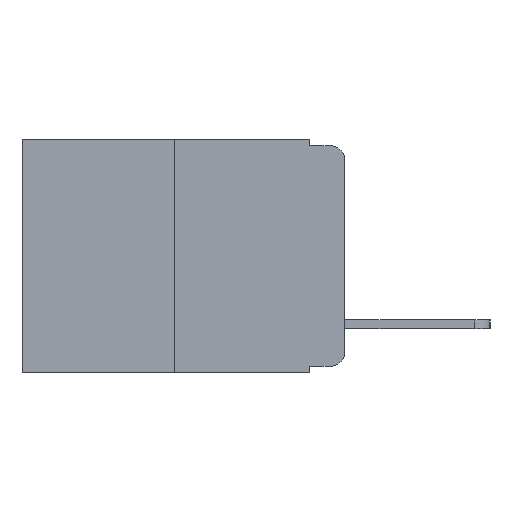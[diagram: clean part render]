
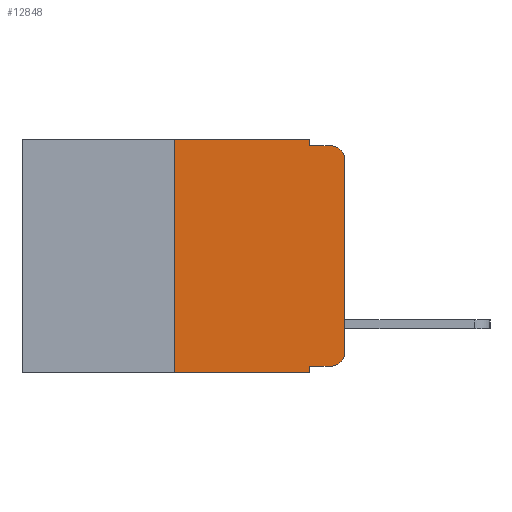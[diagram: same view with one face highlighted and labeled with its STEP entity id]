
A CAD part, left-side view. The second image highlights one B-rep face of the part: STEP entity #12848.
In plain terms, the highlighted planar face has unit normal (-1, 0, 0).
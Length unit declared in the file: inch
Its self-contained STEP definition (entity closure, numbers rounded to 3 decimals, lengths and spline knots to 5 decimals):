
#46 = ORIENTED_EDGE ( 'NONE', *, *, #10113, .T. ) ;
#92 = VECTOR ( 'NONE', #14581, 39.37008 ) ;
#102 = DIRECTION ( 'NONE',  ( 1., 0., 0. ) ) ;
#132 = CARTESIAN_POINT ( 'NONE',  ( 0., 0.02, -0.313 ) ) ;
#219 = VERTEX_POINT ( 'NONE', #14642 ) ;
#473 = CARTESIAN_POINT ( 'NONE',  ( 0., 0., -0.03 ) ) ;
#903 = VECTOR ( 'NONE', #10060, 39.37008 ) ;
#1251 = VERTEX_POINT ( 'NONE', #1979 ) ;
#1410 = EDGE_CURVE ( 'NONE', #9491, #15023, #4073, .T. ) ;
#1529 = DIRECTION ( 'NONE',  ( 0., 0., -1. ) ) ;
#1979 = CARTESIAN_POINT ( 'NONE',  ( 0., 0.25, -0.343 ) ) ;
#2309 = EDGE_CURVE ( 'NONE', #9491, #8995, #4041, .T. ) ;
#2317 = DIRECTION ( 'NONE',  ( 0., -1., 0. ) ) ;
#2526 = FACE_OUTER_BOUND ( 'NONE', #15947, .T. ) ;
#2939 = ORIENTED_EDGE ( 'NONE', *, *, #16074, .T. ) ;
#3181 = EDGE_CURVE ( 'NONE', #1251, #8301, #5237, .T. ) ;
#3269 = AXIS2_PLACEMENT_3D ( 'NONE', #12316, #4678, #13518 ) ;
#3487 = ORIENTED_EDGE ( 'NONE', *, *, #7555, .F. ) ;
#3507 = ORIENTED_EDGE ( 'NONE', *, *, #4931, .F. ) ;
#3775 = LINE ( 'NONE', #3844, #13476 ) ;
#3844 = CARTESIAN_POINT ( 'NONE',  ( 0., 0.051, -0.01 ) ) ;
#4041 = LINE ( 'NONE', #13116, #13716 ) ;
#4073 = LINE ( 'NONE', #10340, #92 ) ;
#4083 = CARTESIAN_POINT ( 'NONE',  ( 0., 0.473, 0. ) ) ;
#4241 = ORIENTED_EDGE ( 'NONE', *, *, #9272, .T. ) ;
#4269 = CIRCLE ( 'NONE', #10270, 0.02 ) ;
#4285 = AXIS2_PLACEMENT_3D ( 'NONE', #4083, #102, #9298 ) ;
#4678 = DIRECTION ( 'NONE',  ( -1., 0., 0. ) ) ;
#4692 = VECTOR ( 'NONE', #2317, 39.37008 ) ;
#4822 = VERTEX_POINT ( 'NONE', #9692 ) ;
#4849 = ORIENTED_EDGE ( 'NONE', *, *, #2309, .F. ) ;
#4856 = CARTESIAN_POINT ( 'NONE',  ( 0., 0.02, -0.01 ) ) ;
#4931 = EDGE_CURVE ( 'NONE', #219, #9879, #4998, .T. ) ;
#4998 = LINE ( 'NONE', #15694, #8429 ) ;
#5237 = LINE ( 'NONE', #15120, #903 ) ;
#5469 = DIRECTION ( 'NONE',  ( 0., -1., 0. ) ) ;
#5485 = ORIENTED_EDGE ( 'NONE', *, *, #16097, .F. ) ;
#5561 = ORIENTED_EDGE ( 'NONE', *, *, #3181, .F. ) ;
#5907 = CARTESIAN_POINT ( 'NONE',  ( 0., 0.02, -0.333 ) ) ;
#6093 = VECTOR ( 'NONE', #5469, 39.37008 ) ;
#6770 = CIRCLE ( 'NONE', #3269, 0.02 ) ;
#7018 = CARTESIAN_POINT ( 'NONE',  ( 0., 0.25, 0. ) ) ;
#7090 = DIRECTION ( 'NONE',  ( 0., 0., -1. ) ) ;
#7145 = CARTESIAN_POINT ( 'NONE',  ( 0., 0.051, -0.01 ) ) ;
#7507 = DIRECTION ( 'NONE',  ( 0., 0., -1. ) ) ;
#7555 = EDGE_CURVE ( 'NONE', #9879, #9377, #3775, .T. ) ;
#7561 = VECTOR ( 'NONE', #8985, 39.37008 ) ;
#7589 = ORIENTED_EDGE ( 'NONE', *, *, #15168, .T. ) ;
#7991 = PLANE ( 'NONE',  #4285 ) ;
#8301 = VERTEX_POINT ( 'NONE', #7018 ) ;
#8429 = VECTOR ( 'NONE', #7090, 39.37008 ) ;
#8985 = DIRECTION ( 'NONE',  ( 0., 0., 1. ) ) ;
#8995 = VERTEX_POINT ( 'NONE', #16280 ) ;
#9272 = EDGE_CURVE ( 'NONE', #13026, #9377, #6770, .T. ) ;
#9298 = DIRECTION ( 'NONE',  ( 0., 0., -1. ) ) ;
#9321 = DIRECTION ( 'NONE',  ( -1., 0., 0. ) ) ;
#9377 = VERTEX_POINT ( 'NONE', #4856 ) ;
#9491 = VERTEX_POINT ( 'NONE', #11477 ) ;
#9535 = LINE ( 'NONE', #14224, #6093 ) ;
#9692 = CARTESIAN_POINT ( 'NONE',  ( 0., 0., -0.313 ) ) ;
#9879 = VERTEX_POINT ( 'NONE', #7145 ) ;
#10060 = DIRECTION ( 'NONE',  ( 0., 0., 1. ) ) ;
#10067 = CARTESIAN_POINT ( 'NONE',  ( 0., 0.473, -0.343 ) ) ;
#10113 = EDGE_CURVE ( 'NONE', #4822, #13026, #10942, .T. ) ;
#10270 = AXIS2_PLACEMENT_3D ( 'NONE', #132, #9321, #1529 ) ;
#10340 = CARTESIAN_POINT ( 'NONE',  ( 0., 0.051, -0.333 ) ) ;
#10807 = ORIENTED_EDGE ( 'NONE', *, *, #1410, .T. ) ;
#10942 = LINE ( 'NONE', #16249, #7561 ) ;
#11477 = CARTESIAN_POINT ( 'NONE',  ( 0., 0.051, -0.333 ) ) ;
#11530 = LINE ( 'NONE', #10067, #4692 ) ;
#11534 = DIRECTION ( 'NONE',  ( 0., -1., 0. ) ) ;
#12316 = CARTESIAN_POINT ( 'NONE',  ( 0., 0.02, -0.03 ) ) ;
#12848 = ADVANCED_FACE ( 'NONE', ( #2526 ), #7991, .F. ) ;
#13026 = VERTEX_POINT ( 'NONE', #473 ) ;
#13116 = CARTESIAN_POINT ( 'NONE',  ( 0., 0.051, 0. ) ) ;
#13476 = VECTOR ( 'NONE', #11534, 39.37008 ) ;
#13518 = DIRECTION ( 'NONE',  ( 0., 0., -1. ) ) ;
#13716 = VECTOR ( 'NONE', #7507, 39.37008 ) ;
#14224 = CARTESIAN_POINT ( 'NONE',  ( 0., 0.473, 0. ) ) ;
#14581 = DIRECTION ( 'NONE',  ( 0., -1., 0. ) ) ;
#14642 = CARTESIAN_POINT ( 'NONE',  ( 0., 0.051, 0. ) ) ;
#15023 = VERTEX_POINT ( 'NONE', #5907 ) ;
#15120 = CARTESIAN_POINT ( 'NONE',  ( 0., 0.25, 0. ) ) ;
#15168 = EDGE_CURVE ( 'NONE', #1251, #8995, #11530, .T. ) ;
#15694 = CARTESIAN_POINT ( 'NONE',  ( 0., 0.051, 0. ) ) ;
#15947 = EDGE_LOOP ( 'NONE', ( #46, #4241, #3487, #3507, #5485, #5561, #7589, #4849, #10807, #2939 ) ) ;
#16074 = EDGE_CURVE ( 'NONE', #15023, #4822, #4269, .T. ) ;
#16097 = EDGE_CURVE ( 'NONE', #8301, #219, #9535, .T. ) ;
#16249 = CARTESIAN_POINT ( 'NONE',  ( 0., 0., 0. ) ) ;
#16280 = CARTESIAN_POINT ( 'NONE',  ( 0., 0.051, -0.343 ) ) ;
